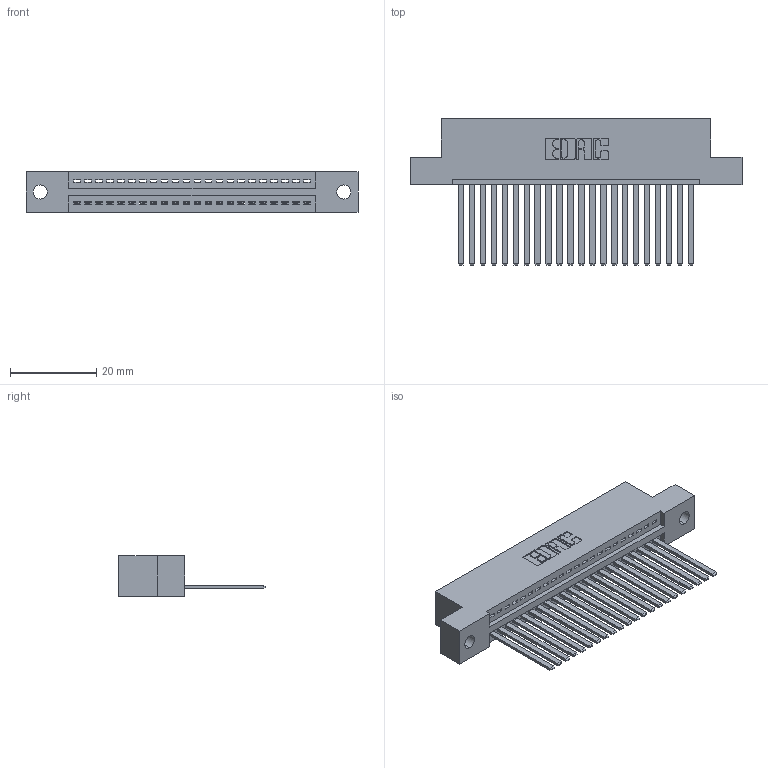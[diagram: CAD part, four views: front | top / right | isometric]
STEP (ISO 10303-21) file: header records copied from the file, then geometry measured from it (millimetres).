
FILE_DESCRIPTION (( 'STEP AP203' ), '1' );
FILE_NAME ('395-022-544-102.STEP', '2019-10-18T03:38:44', ( '' ), ( '' ), 'SwSTEP 2.0', 'SolidWorks 2016', '' );
FILE_SCHEMA (( 'CONFIG_CONTROL_DESIGN' ));
Length unit declared in the file: inch
Products named in the file (3): 345-292-001_345-293-144; 345 Part_Flush Mounting Lugs - 0.128 Dia; 395-022-544-102
Assembly tree (23 placements, depth 2):
  395-022-544-102
    345 Part_Flush Mounting Lugs - 0.128 Dia
    345-292-001_345-293-144  x22
Bounding box: 77.09 x 33.96 x 9.4 mm (x, y, z)
Volume: 7376.3 mm3; surface area: 10024 mm2
Topology: 23 solids, 23 shells, 1270 faces, 3817 edges, 2514 vertices
Faces by surface type: plane 872, cylinder 398
Entity records: 19069 total; most frequent: CARTESIAN_POINT 3310, ORIENTED_EDGE 3266, DIRECTION 2917, EDGE_CURVE 1633, VECTOR 1417, LINE 1417, VERTEX_POINT 1086, AXIS2_PLACEMENT_3D 750
